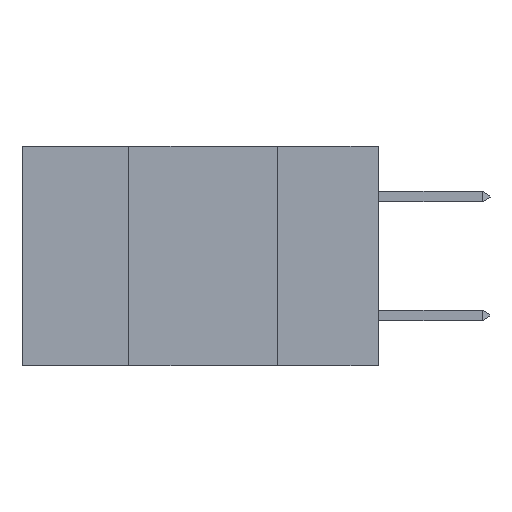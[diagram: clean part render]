
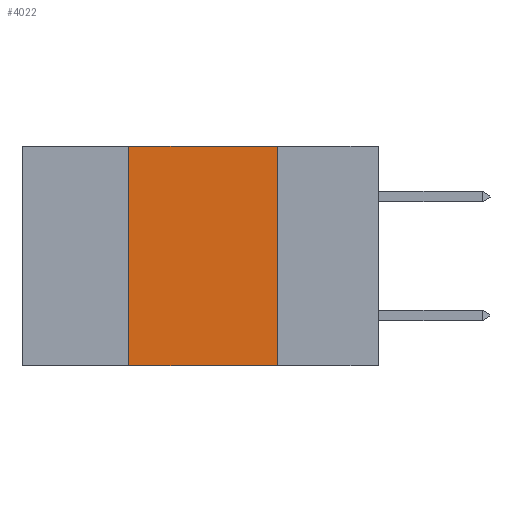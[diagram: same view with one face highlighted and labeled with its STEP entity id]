
A CAD part, left-side view. The second image highlights one B-rep face of the part: STEP entity #4022.
In plain terms, the highlighted planar face has unit normal (-1, 0, 0).
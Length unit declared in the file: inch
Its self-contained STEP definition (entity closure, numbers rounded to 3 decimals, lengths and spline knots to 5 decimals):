
#762 = VERTEX_POINT ( 'NONE', #1143 ) ;
#1143 = CARTESIAN_POINT ( 'NONE',  ( 0., 0.17, -0.37 ) ) ;
#1910 = CARTESIAN_POINT ( 'NONE',  ( 0., 0.6, 0. ) ) ;
#2061 = EDGE_CURVE ( 'NONE', #17543, #7081, #24167, .T. ) ;
#3672 = VERTEX_POINT ( 'NONE', #4881 ) ;
#3821 = VECTOR ( 'NONE', #19625, 39.37008 ) ;
#4015 = DIRECTION ( 'NONE',  ( 1., 0., 0. ) ) ;
#4022 = ADVANCED_FACE ( 'NONE', ( #24094 ), #27917, .F. ) ;
#4881 = CARTESIAN_POINT ( 'NONE',  ( 0., 0.42, -0.37 ) ) ;
#5605 = DIRECTION ( 'NONE',  ( 0., -1., 0. ) ) ;
#6092 = VECTOR ( 'NONE', #15172, 39.37008 ) ;
#7081 = VERTEX_POINT ( 'NONE', #22855 ) ;
#10221 = EDGE_CURVE ( 'NONE', #3672, #17543, #13331, .T. ) ;
#11954 = LINE ( 'NONE', #16563, #17094 ) ;
#12209 = CARTESIAN_POINT ( 'NONE',  ( 0., 0.42, 0. ) ) ;
#13148 = EDGE_CURVE ( 'NONE', #7081, #762, #14815, .T. ) ;
#13162 = CARTESIAN_POINT ( 'NONE',  ( 0., 0.17, 0. ) ) ;
#13331 = LINE ( 'NONE', #12209, #24828 ) ;
#14429 = DIRECTION ( 'NONE',  ( 0., 0., 1. ) ) ;
#14815 = LINE ( 'NONE', #13162, #3821 ) ;
#15172 = DIRECTION ( 'NONE',  ( 0., -1., 0. ) ) ;
#16563 = CARTESIAN_POINT ( 'NONE',  ( 0., 0.6, -0.37 ) ) ;
#17094 = VECTOR ( 'NONE', #5605, 39.37008 ) ;
#17543 = VERTEX_POINT ( 'NONE', #24178 ) ;
#18050 = ORIENTED_EDGE ( 'NONE', *, *, #13148, .F. ) ;
#18173 = ORIENTED_EDGE ( 'NONE', *, *, #18997, .T. ) ;
#18653 = ORIENTED_EDGE ( 'NONE', *, *, #10221, .F. ) ;
#18782 = AXIS2_PLACEMENT_3D ( 'NONE', #21415, #4015, #19348 ) ;
#18997 = EDGE_CURVE ( 'NONE', #3672, #762, #11954, .T. ) ;
#19348 = DIRECTION ( 'NONE',  ( 0., 0., -1. ) ) ;
#19625 = DIRECTION ( 'NONE',  ( 0., 0., -1. ) ) ;
#21231 = ORIENTED_EDGE ( 'NONE', *, *, #2061, .F. ) ;
#21415 = CARTESIAN_POINT ( 'NONE',  ( 0., 0.6, 0. ) ) ;
#22022 = EDGE_LOOP ( 'NONE', ( #18050, #21231, #18653, #18173 ) ) ;
#22855 = CARTESIAN_POINT ( 'NONE',  ( 0., 0.17, 0. ) ) ;
#24094 = FACE_OUTER_BOUND ( 'NONE', #22022, .T. ) ;
#24167 = LINE ( 'NONE', #1910, #6092 ) ;
#24178 = CARTESIAN_POINT ( 'NONE',  ( 0., 0.42, 0. ) ) ;
#24828 = VECTOR ( 'NONE', #14429, 39.37008 ) ;
#27917 = PLANE ( 'NONE',  #18782 ) ;
